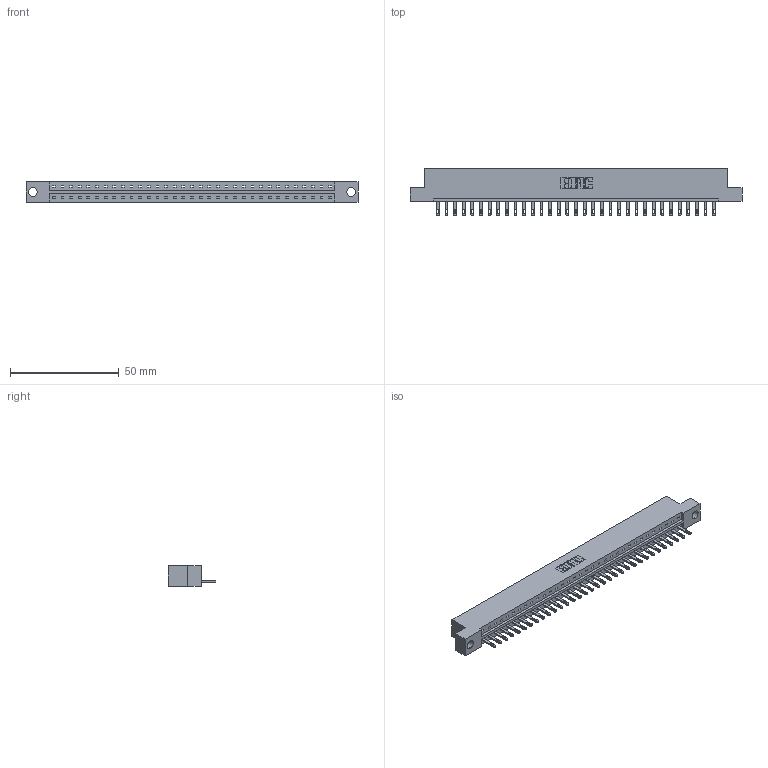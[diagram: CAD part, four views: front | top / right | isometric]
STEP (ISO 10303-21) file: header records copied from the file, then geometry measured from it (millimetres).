
FILE_DESCRIPTION (( 'STEP AP203' ), '1' );
FILE_NAME ('333-033-500-104.STEP', '2018-08-02T20:55:21', ( '' ), ( '' ), 'SwSTEP 2.0', 'SolidWorks 2016', '' );
FILE_SCHEMA (( 'CONFIG_CONTROL_DESIGN' ));
Length unit declared in the file: inch
Products named in the file (3): 333 Part_Flush - .156 Dia - TH; 345-292-001_345-293-100; 333-033-500-104
Assembly tree (34 placements, depth 2):
  333-033-500-104
    333 Part_Flush - .156 Dia - TH
    345-292-001_345-293-100  x33
Bounding box: 152.3 x 21.85 x 9.4 mm (x, y, z)
Volume: 15180.7 mm3; surface area: 16241.9 mm2
Topology: 34 solids, 34 shells, 1896 faces, 5855 edges, 3902 vertices
Faces by surface type: plane 1258, cylinder 638
Entity records: 21271 total; most frequent: CARTESIAN_POINT 3677, ORIENTED_EDGE 3646, DIRECTION 3121, EDGE_CURVE 1823, LINE 1691, VECTOR 1691, VERTEX_POINT 1214, AXIS2_PLACEMENT_3D 715
